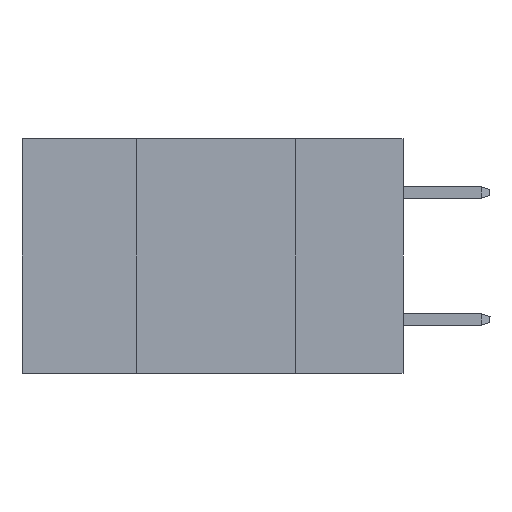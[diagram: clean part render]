
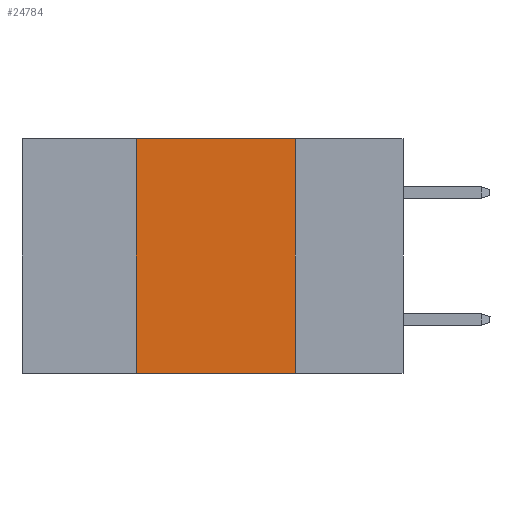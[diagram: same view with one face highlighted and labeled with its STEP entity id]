
A CAD part, left-side view. The second image highlights one B-rep face of the part: STEP entity #24784.
In plain terms, the highlighted planar face has unit normal (-1, 0, 0).
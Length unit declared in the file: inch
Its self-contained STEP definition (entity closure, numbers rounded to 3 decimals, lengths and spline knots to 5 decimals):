
#185 = CARTESIAN_POINT ( 'NONE',  ( 0., 0.42, 0. ) ) ;
#2219 = CARTESIAN_POINT ( 'NONE',  ( 0., 0.17, -0.37 ) ) ;
#5944 = EDGE_CURVE ( 'NONE', #12547, #13737, #13777, .T. ) ;
#8572 = LINE ( 'NONE', #20166, #27533 ) ;
#10051 = EDGE_CURVE ( 'NONE', #32566, #12547, #8572, .T. ) ;
#11867 = DIRECTION ( 'NONE',  ( 0., 0., 1. ) ) ;
#12156 = ORIENTED_EDGE ( 'NONE', *, *, #10051, .F. ) ;
#12316 = CARTESIAN_POINT ( 'NONE',  ( 0., 0.42, -0.37 ) ) ;
#12547 = VERTEX_POINT ( 'NONE', #30712 ) ;
#13123 = EDGE_LOOP ( 'NONE', ( #20155, #12156, #24006, #20377 ) ) ;
#13737 = VERTEX_POINT ( 'NONE', #2219 ) ;
#13777 = LINE ( 'NONE', #26558, #38552 ) ;
#14442 = CARTESIAN_POINT ( 'NONE',  ( 0., 0.42, 0. ) ) ;
#14695 = FACE_OUTER_BOUND ( 'NONE', #13123, .T. ) ;
#15687 = VECTOR ( 'NONE', #11867, 39.37008 ) ;
#16134 = EDGE_CURVE ( 'NONE', #29909, #32566, #27366, .T. ) ;
#17351 = CARTESIAN_POINT ( 'NONE',  ( 0., 0.6, -0.37 ) ) ;
#17937 = DIRECTION ( 'NONE',  ( 0., -1., 0. ) ) ;
#18014 = CARTESIAN_POINT ( 'NONE',  ( 0., 0.6, 0. ) ) ;
#19015 = VECTOR ( 'NONE', #17937, 39.37008 ) ;
#20155 = ORIENTED_EDGE ( 'NONE', *, *, #5944, .F. ) ;
#20166 = CARTESIAN_POINT ( 'NONE',  ( 0., 0.6, 0. ) ) ;
#20377 = ORIENTED_EDGE ( 'NONE', *, *, #28396, .T. ) ;
#23613 = DIRECTION ( 'NONE',  ( 0., 0., -1. ) ) ;
#24006 = ORIENTED_EDGE ( 'NONE', *, *, #16134, .F. ) ;
#24784 = ADVANCED_FACE ( 'NONE', ( #14695 ), #26689, .F. ) ;
#26307 = DIRECTION ( 'NONE',  ( 1., 0., 0. ) ) ;
#26558 = CARTESIAN_POINT ( 'NONE',  ( 0., 0.17, 0. ) ) ;
#26689 = PLANE ( 'NONE',  #31670 ) ;
#27366 = LINE ( 'NONE', #185, #15687 ) ;
#27533 = VECTOR ( 'NONE', #32202, 39.37008 ) ;
#28396 = EDGE_CURVE ( 'NONE', #29909, #13737, #36054, .T. ) ;
#29909 = VERTEX_POINT ( 'NONE', #12316 ) ;
#30712 = CARTESIAN_POINT ( 'NONE',  ( 0., 0.17, 0. ) ) ;
#31670 = AXIS2_PLACEMENT_3D ( 'NONE', #18014, #26307, #32421 ) ;
#32202 = DIRECTION ( 'NONE',  ( 0., -1., 0. ) ) ;
#32421 = DIRECTION ( 'NONE',  ( 0., 0., -1. ) ) ;
#32566 = VERTEX_POINT ( 'NONE', #14442 ) ;
#36054 = LINE ( 'NONE', #17351, #19015 ) ;
#38552 = VECTOR ( 'NONE', #23613, 39.37008 ) ;
